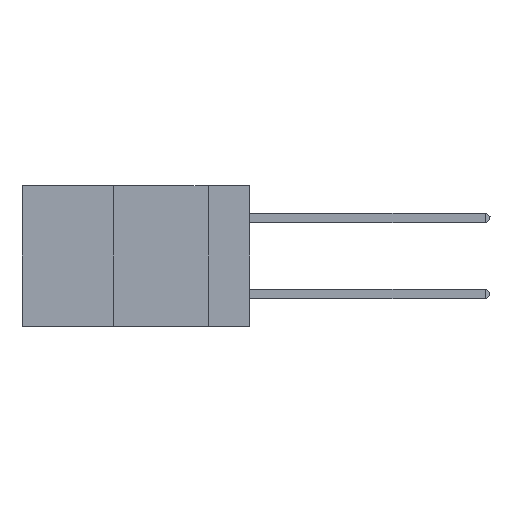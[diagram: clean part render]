
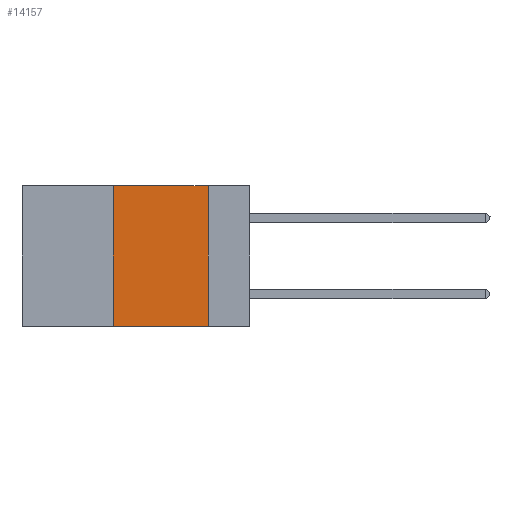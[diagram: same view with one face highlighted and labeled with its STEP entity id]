
A CAD part, left-side view. The second image highlights one B-rep face of the part: STEP entity #14157.
In plain terms, the highlighted planar face has unit normal (-1, 0, 0).
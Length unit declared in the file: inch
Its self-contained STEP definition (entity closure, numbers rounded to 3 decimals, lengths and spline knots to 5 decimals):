
#1883 = VERTEX_POINT ( 'NONE', #37607 ) ;
#3206 = CARTESIAN_POINT ( 'NONE',  ( 0., 0.6, 0. ) ) ;
#4641 = VERTEX_POINT ( 'NONE', #33416 ) ;
#4966 = LINE ( 'NONE', #22139, #31622 ) ;
#5300 = LINE ( 'NONE', #30618, #31949 ) ;
#6778 = DIRECTION ( 'NONE',  ( 0., 0., -1. ) ) ;
#8391 = VERTEX_POINT ( 'NONE', #33975 ) ;
#9091 = ORIENTED_EDGE ( 'NONE', *, *, #23086, .T. ) ;
#9376 = CARTESIAN_POINT ( 'NONE',  ( 0., 0.11, -0.37 ) ) ;
#13100 = DIRECTION ( 'NONE',  ( 0., -1., 0. ) ) ;
#13508 = DIRECTION ( 'NONE',  ( 0., 0., 1. ) ) ;
#13674 = PLANE ( 'NONE',  #20583 ) ;
#14157 = ADVANCED_FACE ( 'NONE', ( #42321 ), #13674, .F. ) ;
#14338 = VECTOR ( 'NONE', #13100, 39.37008 ) ;
#14439 = EDGE_CURVE ( 'NONE', #1883, #16673, #4966, .T. ) ;
#15642 = EDGE_LOOP ( 'NONE', ( #40394, #33440, #16174, #9091 ) ) ;
#16174 = ORIENTED_EDGE ( 'NONE', *, *, #34643, .F. ) ;
#16673 = VERTEX_POINT ( 'NONE', #9376 ) ;
#17008 = CARTESIAN_POINT ( 'NONE',  ( 0., 0.6, -0.37 ) ) ;
#18294 = EDGE_CURVE ( 'NONE', #8391, #1883, #24655, .T. ) ;
#20583 = AXIS2_PLACEMENT_3D ( 'NONE', #3206, #27626, #6778 ) ;
#22139 = CARTESIAN_POINT ( 'NONE',  ( 0., 0.11, 0. ) ) ;
#23086 = EDGE_CURVE ( 'NONE', #4641, #16673, #35423, .T. ) ;
#24655 = LINE ( 'NONE', #43914, #14338 ) ;
#25632 = DIRECTION ( 'NONE',  ( 0., 0., -1. ) ) ;
#27313 = DIRECTION ( 'NONE',  ( 0., -1., 0. ) ) ;
#27626 = DIRECTION ( 'NONE',  ( 1., 0., 0. ) ) ;
#30618 = CARTESIAN_POINT ( 'NONE',  ( 0., 0.36, 0. ) ) ;
#31622 = VECTOR ( 'NONE', #25632, 39.37008 ) ;
#31949 = VECTOR ( 'NONE', #13508, 39.37008 ) ;
#33416 = CARTESIAN_POINT ( 'NONE',  ( 0., 0.36, -0.37 ) ) ;
#33440 = ORIENTED_EDGE ( 'NONE', *, *, #18294, .F. ) ;
#33975 = CARTESIAN_POINT ( 'NONE',  ( 0., 0.36, 0. ) ) ;
#34643 = EDGE_CURVE ( 'NONE', #4641, #8391, #5300, .T. ) ;
#35423 = LINE ( 'NONE', #17008, #44524 ) ;
#37607 = CARTESIAN_POINT ( 'NONE',  ( 0., 0.11, 0. ) ) ;
#40394 = ORIENTED_EDGE ( 'NONE', *, *, #14439, .F. ) ;
#42321 = FACE_OUTER_BOUND ( 'NONE', #15642, .T. ) ;
#43914 = CARTESIAN_POINT ( 'NONE',  ( 0., 0.6, 0. ) ) ;
#44524 = VECTOR ( 'NONE', #27313, 39.37008 ) ;
